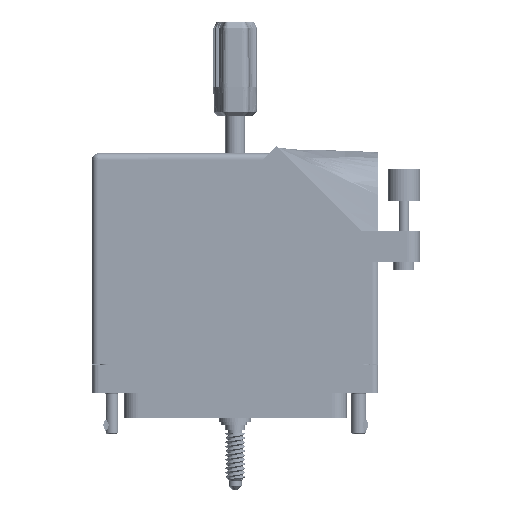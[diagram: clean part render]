
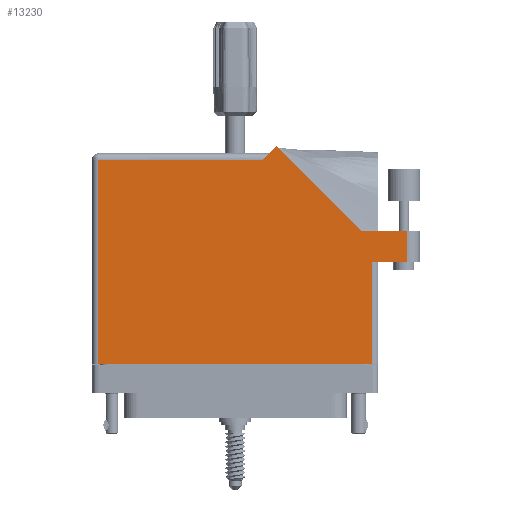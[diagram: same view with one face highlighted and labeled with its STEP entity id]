
A CAD part, front view. The second image highlights one B-rep face of the part: STEP entity #13230.
In plain terms, the highlighted face is planar.
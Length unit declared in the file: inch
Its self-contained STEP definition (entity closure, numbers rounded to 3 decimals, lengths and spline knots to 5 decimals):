
#157 = LINE ( 'NONE', #52734, #43558 ) ;
#765 = VERTEX_POINT ( 'NONE', #22717 ) ;
#3635 = LINE ( 'NONE', #74065, #103036 ) ;
#5992 = VECTOR ( 'NONE', #71236, 39.37008 ) ;
#6885 = CARTESIAN_POINT ( 'NONE',  ( -1.3155, -0.1, 0.765 ) ) ;
#12773 = ORIENTED_EDGE ( 'NONE', *, *, #105521, .T. ) ;
#12929 = CARTESIAN_POINT ( 'NONE',  ( -1.3155, 1.868, 0.765 ) ) ;
#13230 = ADVANCED_FACE ( 'NONE', ( #89173 ), #26300, .F. ) ;
#13303 = VERTEX_POINT ( 'NONE', #60108 ) ;
#14465 = DIRECTION ( 'NONE',  ( 1., 0., 0. ) ) ;
#14749 = CARTESIAN_POINT ( 'NONE',  ( -1.3775, 1.868, 0.765 ) ) ;
#14921 = VECTOR ( 'NONE', #76079, 39.37008 ) ;
#14953 = CARTESIAN_POINT ( 'NONE',  ( 1.6525, 1.187, 0.765 ) ) ;
#17350 = EDGE_CURVE ( 'NONE', #73865, #13303, #157, .T. ) ;
#18326 = VERTEX_POINT ( 'NONE', #12929 ) ;
#18684 = LINE ( 'NONE', #38980, #63398 ) ;
#19844 = ORIENTED_EDGE ( 'NONE', *, *, #50702, .T. ) ;
#20938 = DIRECTION ( 'NONE',  ( 0., 1., 0. ) ) ;
#20941 = EDGE_CURVE ( 'NONE', #765, #41838, #24714, .T. ) ;
#21384 = LINE ( 'NONE', #62293, #5992 ) ;
#22717 = CARTESIAN_POINT ( 'NONE',  ( 1.3155, 0.88, 0.765 ) ) ;
#23896 = EDGE_CURVE ( 'NONE', #18326, #107652, #18684, .T. ) ;
#24714 = LINE ( 'NONE', #93357, #14921 ) ;
#26016 = AXIS2_PLACEMENT_3D ( 'NONE', #62211, #36382, #97915 ) ;
#26300 = PLANE ( 'NONE',  #26016 ) ;
#26486 = VERTEX_POINT ( 'NONE', #44904 ) ;
#29748 = EDGE_CURVE ( 'NONE', #107652, #26486, #86334, .T. ) ;
#29814 = ORIENTED_EDGE ( 'NONE', *, *, #75724, .T. ) ;
#31213 = VECTOR ( 'NONE', #50117, 39.37008 ) ;
#34087 = DIRECTION ( 'NONE',  ( 0., 1., 0. ) ) ;
#36382 = DIRECTION ( 'NONE',  ( 0., 0., -1. ) ) ;
#38682 = VECTOR ( 'NONE', #14465, 39.37008 ) ;
#38980 = CARTESIAN_POINT ( 'NONE',  ( -1.3155, -0.1, 0.765 ) ) ;
#41178 = CARTESIAN_POINT ( 'NONE',  ( 0.3275, 1.93, 0.765 ) ) ;
#41838 = VERTEX_POINT ( 'NONE', #100013 ) ;
#42940 = ORIENTED_EDGE ( 'NONE', *, *, #17350, .T. ) ;
#43558 = VECTOR ( 'NONE', #60586, 39.37008 ) ;
#43737 = ORIENTED_EDGE ( 'NONE', *, *, #86053, .T. ) ;
#44904 = CARTESIAN_POINT ( 'NONE',  ( 1.3155, -0.1, 0.765 ) ) ;
#48478 = EDGE_LOOP ( 'NONE', ( #53909, #12773, #29814, #42940, #43737, #19844, #53474, #51099, #81990 ) ) ;
#50117 = DIRECTION ( 'NONE',  ( -0.707, -0.707, 0. ) ) ;
#50616 = VERTEX_POINT ( 'NONE', #102052 ) ;
#50702 = EDGE_CURVE ( 'NONE', #52774, #18326, #103246, .T. ) ;
#51099 = ORIENTED_EDGE ( 'NONE', *, *, #29748, .T. ) ;
#52734 = CARTESIAN_POINT ( 'NONE',  ( 1.21192, 1.187, 0.765 ) ) ;
#52774 = VERTEX_POINT ( 'NONE', #107832 ) ;
#53474 = ORIENTED_EDGE ( 'NONE', *, *, #23896, .T. ) ;
#53909 = ORIENTED_EDGE ( 'NONE', *, *, #20941, .T. ) ;
#57685 = VECTOR ( 'NONE', #34087, 39.37008 ) ;
#60108 = CARTESIAN_POINT ( 'NONE',  ( 0.39821, 2.00071, 0.765 ) ) ;
#60586 = DIRECTION ( 'NONE',  ( -0.707, 0.707, 0. ) ) ;
#62211 = CARTESIAN_POINT ( 'NONE',  ( -1.3775, 1.93, 0.765 ) ) ;
#62293 = CARTESIAN_POINT ( 'NONE',  ( 1.7775, 1.187, 0.765 ) ) ;
#63398 = VECTOR ( 'NONE', #93036, 39.37008 ) ;
#71236 = DIRECTION ( 'NONE',  ( -1., 0., 0. ) ) ;
#73865 = VERTEX_POINT ( 'NONE', #75308 ) ;
#74065 = CARTESIAN_POINT ( 'NONE',  ( 1.3155, 0.88, 0.765 ) ) ;
#75308 = CARTESIAN_POINT ( 'NONE',  ( 1.21192, 1.187, 0.765 ) ) ;
#75724 = EDGE_CURVE ( 'NONE', #50616, #73865, #21384, .T. ) ;
#76079 = DIRECTION ( 'NONE',  ( 1., 0., 0. ) ) ;
#81990 = ORIENTED_EDGE ( 'NONE', *, *, #91381, .T. ) ;
#84454 = LINE ( 'NONE', #41178, #31213 ) ;
#84902 = CARTESIAN_POINT ( 'NONE',  ( -1.3775, -0.1, 0.765 ) ) ;
#86053 = EDGE_CURVE ( 'NONE', #13303, #52774, #84454, .T. ) ;
#86334 = LINE ( 'NONE', #84902, #38682 ) ;
#89173 = FACE_OUTER_BOUND ( 'NONE', #48478, .T. ) ;
#89969 = LINE ( 'NONE', #14953, #57685 ) ;
#91381 = EDGE_CURVE ( 'NONE', #26486, #765, #3635, .T. ) ;
#93036 = DIRECTION ( 'NONE',  ( 0., -1., 0. ) ) ;
#93357 = CARTESIAN_POINT ( 'NONE',  ( 1.3775, 0.88, 0.765 ) ) ;
#95373 = DIRECTION ( 'NONE',  ( -1., 0., 0. ) ) ;
#97915 = DIRECTION ( 'NONE',  ( -1., 0., 0. ) ) ;
#100013 = CARTESIAN_POINT ( 'NONE',  ( 1.6525, 0.88, 0.765 ) ) ;
#102052 = CARTESIAN_POINT ( 'NONE',  ( 1.6525, 1.187, 0.765 ) ) ;
#103036 = VECTOR ( 'NONE', #20938, 39.37008 ) ;
#103246 = LINE ( 'NONE', #14749, #112848 ) ;
#105521 = EDGE_CURVE ( 'NONE', #41838, #50616, #89969, .T. ) ;
#107652 = VERTEX_POINT ( 'NONE', #6885 ) ;
#107832 = CARTESIAN_POINT ( 'NONE',  ( 0.2655, 1.868, 0.765 ) ) ;
#112848 = VECTOR ( 'NONE', #95373, 39.37008 ) ;
